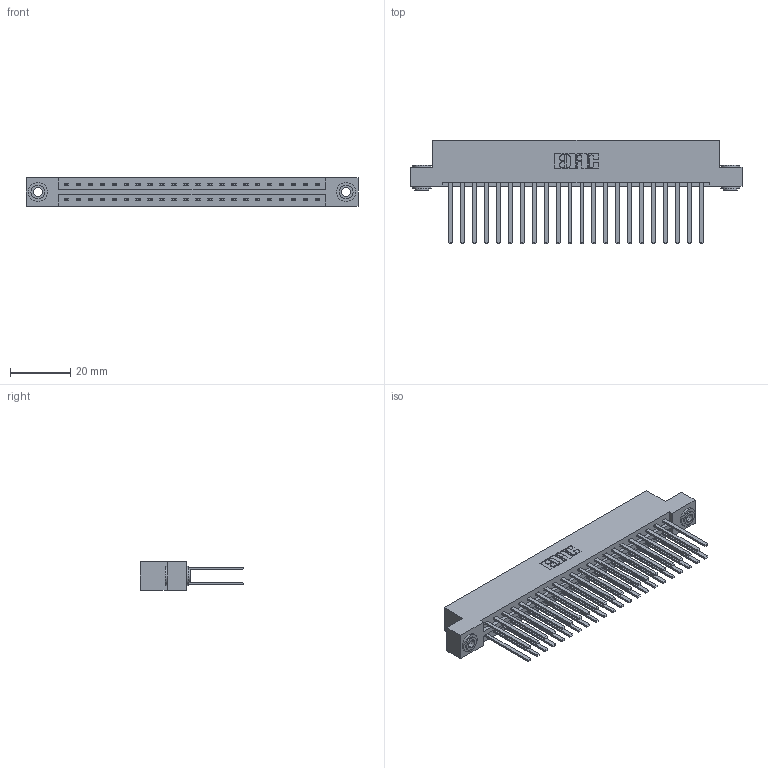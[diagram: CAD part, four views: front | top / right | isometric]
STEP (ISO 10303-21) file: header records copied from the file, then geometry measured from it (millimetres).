
FILE_DESCRIPTION (( 'STEP AP203' ), '1' );
FILE_NAME ('387-044-544-203.STEP', '2019-10-18T06:01:05', ( '' ), ( '' ), 'SwSTEP 2.0', 'SolidWorks 2016', '' );
FILE_SCHEMA (( 'CONFIG_CONTROL_DESIGN' ));
Length unit declared in the file: inch
Products named in the file (4): 345-292-001_345-293-144; 387-044-544-203; 345-250-002_345-250-002-102; 337 Part_Flush Mounting Lugs - 0.156 Dia-TH
Assembly tree (47 placements, depth 2):
  387-044-544-203
    337 Part_Flush Mounting Lugs - 0.156 Dia-TH
    345-292-001_345-293-144  x44
    345-250-002_345-250-002-102  x2
Bounding box: 110.19 x 34.3 x 9.4 mm (x, y, z)
Volume: 11982.2 mm3; surface area: 15590.9 mm2
Topology: 47 solids, 47 shells, 2264 faces, 6679 edges, 4390 vertices
Faces by surface type: plane 1576, cylinder 680, cone 8
Entity records: 20110 total; most frequent: CARTESIAN_POINT 3377, ORIENTED_EDGE 3306, DIRECTION 2939, EDGE_CURVE 1653, VECTOR 1505, LINE 1505, VERTEX_POINT 1098, AXIS2_PLACEMENT_3D 717
